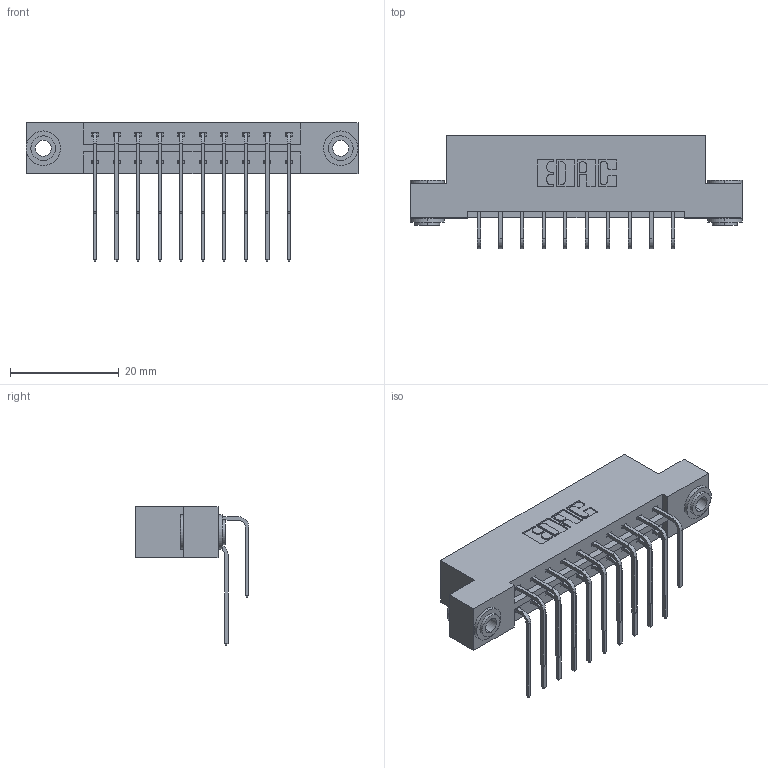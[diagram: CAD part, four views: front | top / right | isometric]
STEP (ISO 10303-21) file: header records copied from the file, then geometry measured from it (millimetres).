
FILE_DESCRIPTION (( 'STEP AP203' ), '1' );
FILE_NAME ('833-020-559-203.STEP', '2020-06-01T14:09:43', ( '' ), ( '' ), 'SwSTEP 2.0', 'SolidWorks 2020', '' );
FILE_SCHEMA (( 'CONFIG_CONTROL_DESIGN' ));
Length unit declared in the file: inch
Products named in the file (5): 833 Part_Flush - .156 Dia - TH; 833-020-559-203; 345-292-001_559 Tail - 2; 345-250-002_345-250-002-102; 345-292-001_558 559 Tail - 1
Assembly tree (23 placements, depth 2):
  833-020-559-203
    833 Part_Flush - .156 Dia - TH
    345-292-001_558 559 Tail - 1  x10
    345-292-001_559 Tail - 2  x10
    345-250-002_345-250-002-102  x2
Bounding box: 61.16 x 20.9 x 25.53 mm (x, y, z)
Volume: 6079.9 mm3; surface area: 7639.7 mm2
Topology: 23 solids, 23 shells, 1232 faces, 3607 edges, 2374 vertices
Faces by surface type: plane 840, cylinder 384, cone 8
Entity records: 13006 total; most frequent: CARTESIAN_POINT 2220, ORIENTED_EDGE 2098, DIRECTION 1967, EDGE_CURVE 1049, LINE 857, VECTOR 857, VERTEX_POINT 694, AXIS2_PLACEMENT_3D 555
